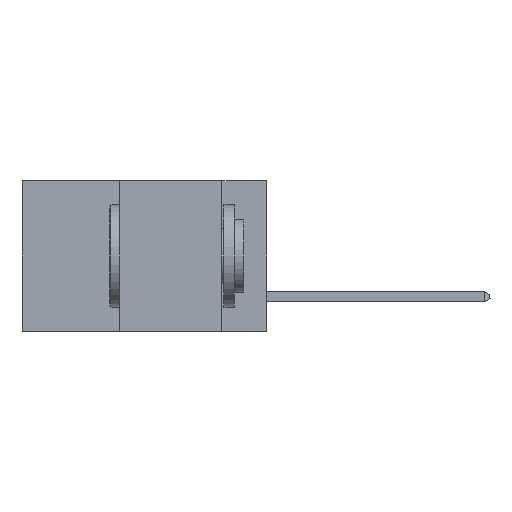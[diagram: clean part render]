
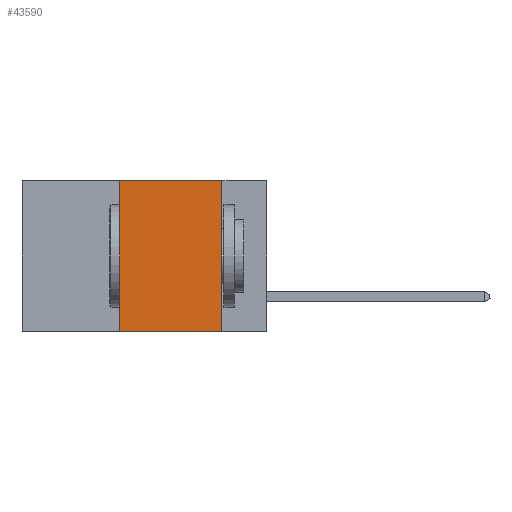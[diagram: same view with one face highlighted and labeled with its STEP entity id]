
A CAD part, left-side view. The second image highlights one B-rep face of the part: STEP entity #43590.
In plain terms, the highlighted planar face has unit normal (-1, 0, 0).
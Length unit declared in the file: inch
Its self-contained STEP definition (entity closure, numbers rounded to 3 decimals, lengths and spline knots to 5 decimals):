
#1554 = EDGE_CURVE ( 'NONE', #18867, #40467, #23181, .T. ) ;
#4206 = CARTESIAN_POINT ( 'NONE',  ( 0., 0.36, 0. ) ) ;
#4469 = ORIENTED_EDGE ( 'NONE', *, *, #1554, .F. ) ;
#4549 = DIRECTION ( 'NONE',  ( 0., 0., -1. ) ) ;
#5196 = EDGE_LOOP ( 'NONE', ( #4469, #12974, #30276, #33047 ) ) ;
#6720 = VECTOR ( 'NONE', #4549, 39.37008 ) ;
#7905 = VECTOR ( 'NONE', #48798, 39.37008 ) ;
#8727 = VERTEX_POINT ( 'NONE', #41190 ) ;
#9078 = FACE_OUTER_BOUND ( 'NONE', #5196, .T. ) ;
#11847 = VERTEX_POINT ( 'NONE', #4206 ) ;
#12974 = ORIENTED_EDGE ( 'NONE', *, *, #21308, .F. ) ;
#16101 = CARTESIAN_POINT ( 'NONE',  ( 0., 0.11, 0. ) ) ;
#17419 = CARTESIAN_POINT ( 'NONE',  ( 0., 0.36, 0. ) ) ;
#18867 = VERTEX_POINT ( 'NONE', #38779 ) ;
#20248 = VECTOR ( 'NONE', #25409, 39.37008 ) ;
#21308 = EDGE_CURVE ( 'NONE', #11847, #18867, #29227, .T. ) ;
#21734 = DIRECTION ( 'NONE',  ( 1., 0., 0. ) ) ;
#22529 = DIRECTION ( 'NONE',  ( 0., -1., 0. ) ) ;
#23181 = LINE ( 'NONE', #16101, #6720 ) ;
#25409 = DIRECTION ( 'NONE',  ( 0., 0., 1. ) ) ;
#28184 = AXIS2_PLACEMENT_3D ( 'NONE', #44988, #21734, #48886 ) ;
#29227 = LINE ( 'NONE', #33380, #7905 ) ;
#30241 = CARTESIAN_POINT ( 'NONE',  ( 0., 0.11, -0.37 ) ) ;
#30276 = ORIENTED_EDGE ( 'NONE', *, *, #45881, .F. ) ;
#31518 = EDGE_CURVE ( 'NONE', #8727, #40467, #50130, .T. ) ;
#33047 = ORIENTED_EDGE ( 'NONE', *, *, #31518, .T. ) ;
#33125 = PLANE ( 'NONE',  #28184 ) ;
#33380 = CARTESIAN_POINT ( 'NONE',  ( 0., 0.6, 0. ) ) ;
#36761 = VECTOR ( 'NONE', #22529, 39.37008 ) ;
#38779 = CARTESIAN_POINT ( 'NONE',  ( 0., 0.11, 0. ) ) ;
#40467 = VERTEX_POINT ( 'NONE', #30241 ) ;
#41190 = CARTESIAN_POINT ( 'NONE',  ( 0., 0.36, -0.37 ) ) ;
#43590 = ADVANCED_FACE ( 'NONE', ( #9078 ), #33125, .F. ) ;
#44227 = CARTESIAN_POINT ( 'NONE',  ( 0., 0.6, -0.37 ) ) ;
#44988 = CARTESIAN_POINT ( 'NONE',  ( 0., 0.6, 0. ) ) ;
#45881 = EDGE_CURVE ( 'NONE', #8727, #11847, #47562, .T. ) ;
#47562 = LINE ( 'NONE', #17419, #20248 ) ;
#48798 = DIRECTION ( 'NONE',  ( 0., -1., 0. ) ) ;
#48886 = DIRECTION ( 'NONE',  ( 0., 0., -1. ) ) ;
#50130 = LINE ( 'NONE', #44227, #36761 ) ;
